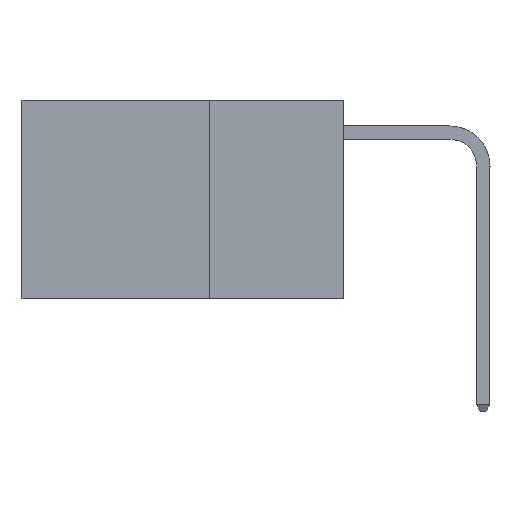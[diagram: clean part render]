
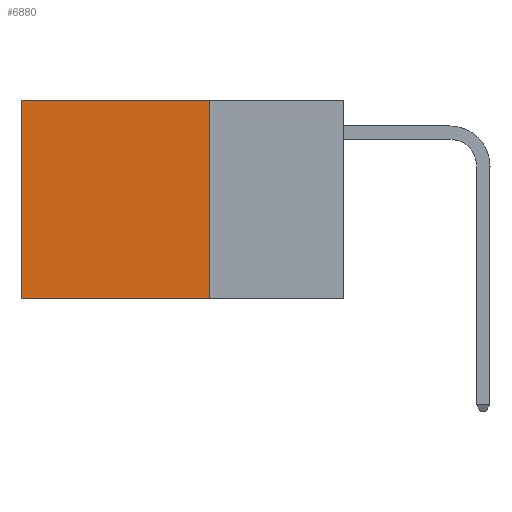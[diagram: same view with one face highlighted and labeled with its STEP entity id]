
A CAD part, left-side view. The second image highlights one B-rep face of the part: STEP entity #6880.
In plain terms, the highlighted planar face has unit normal (-1, 0, 0).
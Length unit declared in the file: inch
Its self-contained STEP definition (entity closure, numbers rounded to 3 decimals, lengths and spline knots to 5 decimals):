
#223 = DIRECTION ( 'NONE',  ( 1., 0., 0. ) ) ;
#957 = EDGE_LOOP ( 'NONE', ( #14054, #3262, #4235, #3418 ) ) ;
#969 = CARTESIAN_POINT ( 'NONE',  ( 0.2625, 0.25, 0. ) ) ;
#1254 = EDGE_CURVE ( 'NONE', #8683, #1837, #5089, .T. ) ;
#1266 = LINE ( 'NONE', #6836, #12626 ) ;
#1431 = CARTESIAN_POINT ( 'NONE',  ( 0.2625, 0.6, 0. ) ) ;
#1837 = VERTEX_POINT ( 'NONE', #11198 ) ;
#2747 = FACE_OUTER_BOUND ( 'NONE', #957, .T. ) ;
#2955 = VERTEX_POINT ( 'NONE', #14143 ) ;
#3262 = ORIENTED_EDGE ( 'NONE', *, *, #11175, .F. ) ;
#3418 = ORIENTED_EDGE ( 'NONE', *, *, #13532, .T. ) ;
#3649 = PLANE ( 'NONE',  #8983 ) ;
#3712 = DIRECTION ( 'NONE',  ( 0., 0., -1. ) ) ;
#4235 = ORIENTED_EDGE ( 'NONE', *, *, #1254, .F. ) ;
#4670 = DIRECTION ( 'NONE',  ( 0., 1., 0. ) ) ;
#5089 = LINE ( 'NONE', #8076, #8014 ) ;
#6231 = EDGE_CURVE ( 'NONE', #2955, #11235, #9921, .T. ) ;
#6836 = CARTESIAN_POINT ( 'NONE',  ( 0.2625, 0.25, 0. ) ) ;
#6880 = ADVANCED_FACE ( 'NONE', ( #2747 ), #3649, .F. ) ;
#6967 = CARTESIAN_POINT ( 'NONE',  ( 0.2625, 0.25, 0. ) ) ;
#8014 = VECTOR ( 'NONE', #3712, 39.37008 ) ;
#8064 = DIRECTION ( 'NONE',  ( 0., 0., -1. ) ) ;
#8076 = CARTESIAN_POINT ( 'NONE',  ( 0.2625, 0.25, 0. ) ) ;
#8683 = VERTEX_POINT ( 'NONE', #969 ) ;
#8900 = DIRECTION ( 'NONE',  ( 0., 1., 0. ) ) ;
#8983 = AXIS2_PLACEMENT_3D ( 'NONE', #6967, #223, #8064 ) ;
#8995 = CARTESIAN_POINT ( 'NONE',  ( 0.2625, 0.6, -0.37 ) ) ;
#9175 = DIRECTION ( 'NONE',  ( 0., 0., -1. ) ) ;
#9921 = LINE ( 'NONE', #1431, #13091 ) ;
#11175 = EDGE_CURVE ( 'NONE', #1837, #11235, #13982, .T. ) ;
#11198 = CARTESIAN_POINT ( 'NONE',  ( 0.2625, 0.25, -0.37 ) ) ;
#11203 = VECTOR ( 'NONE', #8900, 39.37008 ) ;
#11235 = VERTEX_POINT ( 'NONE', #8995 ) ;
#12626 = VECTOR ( 'NONE', #4670, 39.37008 ) ;
#13091 = VECTOR ( 'NONE', #9175, 39.37008 ) ;
#13148 = CARTESIAN_POINT ( 'NONE',  ( 0.2625, 0.25, -0.37 ) ) ;
#13532 = EDGE_CURVE ( 'NONE', #8683, #2955, #1266, .T. ) ;
#13982 = LINE ( 'NONE', #13148, #11203 ) ;
#14054 = ORIENTED_EDGE ( 'NONE', *, *, #6231, .T. ) ;
#14143 = CARTESIAN_POINT ( 'NONE',  ( 0.2625, 0.6, 0. ) ) ;
